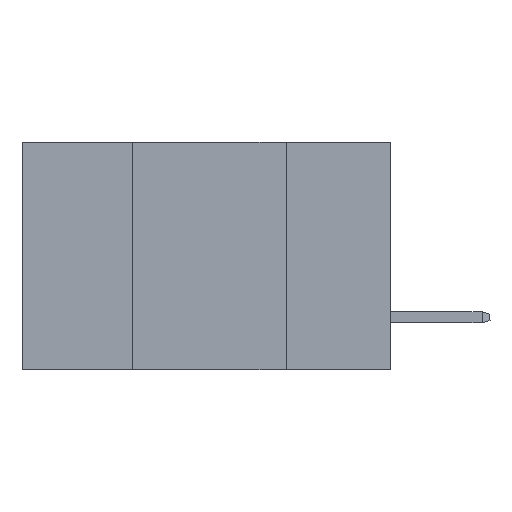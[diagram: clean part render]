
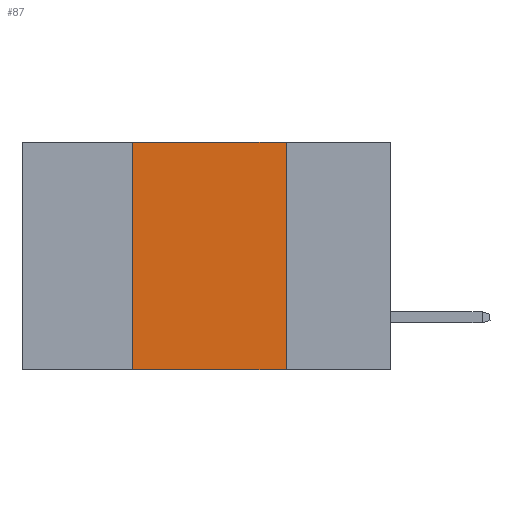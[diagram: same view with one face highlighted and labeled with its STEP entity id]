
A CAD part, left-side view. The second image highlights one B-rep face of the part: STEP entity #87.
In plain terms, the highlighted planar face has unit normal (-1, 0, 0).
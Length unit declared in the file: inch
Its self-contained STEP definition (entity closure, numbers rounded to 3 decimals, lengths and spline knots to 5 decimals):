
#87 = ADVANCED_FACE ( 'NONE', ( #7706 ), #6531, .F. ) ;
#448 = CARTESIAN_POINT ( 'NONE',  ( 0., 0.6, -0.37 ) ) ;
#483 = DIRECTION ( 'NONE',  ( 0., 0., -1. ) ) ;
#1116 = CARTESIAN_POINT ( 'NONE',  ( 0., 0.6, 0. ) ) ;
#1213 = CARTESIAN_POINT ( 'NONE',  ( 0., 0.17, 0. ) ) ;
#1478 = DIRECTION ( 'NONE',  ( 0., 0., -1. ) ) ;
#1685 = DIRECTION ( 'NONE',  ( 0., -1., 0. ) ) ;
#1904 = CARTESIAN_POINT ( 'NONE',  ( 0., 0.17, 0. ) ) ;
#1914 = VERTEX_POINT ( 'NONE', #2006 ) ;
#2006 = CARTESIAN_POINT ( 'NONE',  ( 0., 0.17, -0.37 ) ) ;
#2218 = VERTEX_POINT ( 'NONE', #3016 ) ;
#2465 = EDGE_CURVE ( 'NONE', #7728, #1914, #5050, .T. ) ;
#2772 = EDGE_CURVE ( 'NONE', #2218, #7712, #9566, .T. ) ;
#2974 = DIRECTION ( 'NONE',  ( 0., -1., 0. ) ) ;
#3000 = EDGE_CURVE ( 'NONE', #7712, #1914, #5347, .T. ) ;
#3016 = CARTESIAN_POINT ( 'NONE',  ( 0., 0.42, 0. ) ) ;
#3027 = ORIENTED_EDGE ( 'NONE', *, *, #3000, .F. ) ;
#3080 = VECTOR ( 'NONE', #4134, 39.37008 ) ;
#3392 = EDGE_LOOP ( 'NONE', ( #3027, #3415, #5394, #5149 ) ) ;
#3415 = ORIENTED_EDGE ( 'NONE', *, *, #2772, .F. ) ;
#3541 = DIRECTION ( 'NONE',  ( 1., 0., 0. ) ) ;
#3570 = VECTOR ( 'NONE', #2974, 39.37008 ) ;
#4101 = AXIS2_PLACEMENT_3D ( 'NONE', #6770, #3541, #1478 ) ;
#4134 = DIRECTION ( 'NONE',  ( 0., 0., 1. ) ) ;
#5050 = LINE ( 'NONE', #448, #3570 ) ;
#5149 = ORIENTED_EDGE ( 'NONE', *, *, #2465, .T. ) ;
#5347 = LINE ( 'NONE', #1213, #8810 ) ;
#5394 = ORIENTED_EDGE ( 'NONE', *, *, #9260, .F. ) ;
#6254 = CARTESIAN_POINT ( 'NONE',  ( 0., 0.42, 0. ) ) ;
#6531 = PLANE ( 'NONE',  #4101 ) ;
#6770 = CARTESIAN_POINT ( 'NONE',  ( 0., 0.6, 0. ) ) ;
#6860 = LINE ( 'NONE', #6254, #3080 ) ;
#7706 = FACE_OUTER_BOUND ( 'NONE', #3392, .T. ) ;
#7712 = VERTEX_POINT ( 'NONE', #1904 ) ;
#7728 = VERTEX_POINT ( 'NONE', #8809 ) ;
#7997 = VECTOR ( 'NONE', #1685, 39.37008 ) ;
#8809 = CARTESIAN_POINT ( 'NONE',  ( 0., 0.42, -0.37 ) ) ;
#8810 = VECTOR ( 'NONE', #483, 39.37008 ) ;
#9260 = EDGE_CURVE ( 'NONE', #7728, #2218, #6860, .T. ) ;
#9566 = LINE ( 'NONE', #1116, #7997 ) ;
